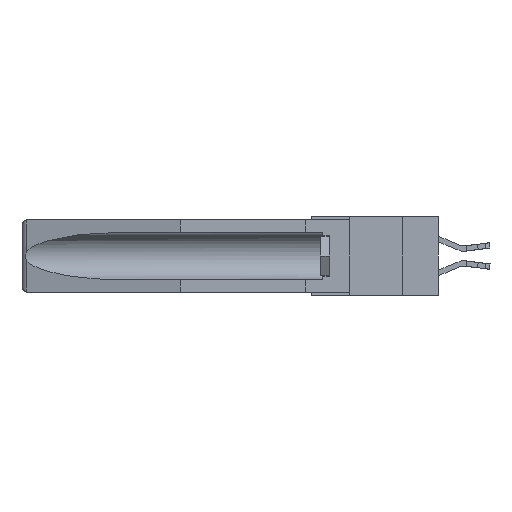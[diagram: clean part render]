
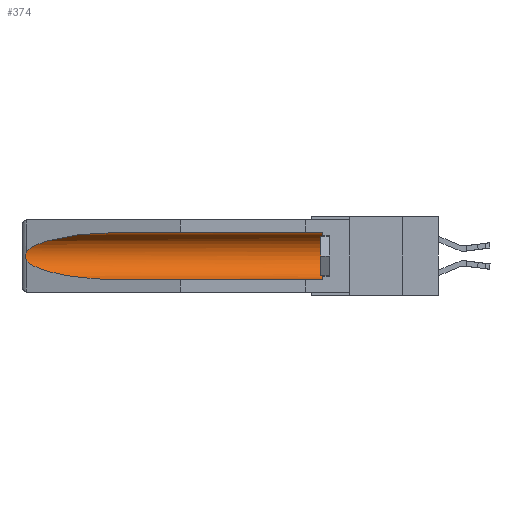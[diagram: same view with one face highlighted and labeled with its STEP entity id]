
A CAD part, left-side view. The second image highlights one B-rep face of the part: STEP entity #374.
In plain terms, the highlighted cylindrical face has radius 2.857 mm (diameter 5.715 mm), a partial arc.
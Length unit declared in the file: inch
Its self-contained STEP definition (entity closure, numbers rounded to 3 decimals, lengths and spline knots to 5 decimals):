
#374 = ADVANCED_FACE ( 'NONE', ( #2719 ), #3018, .F. ) ;
#740 = CARTESIAN_POINT ( 'NONE',  ( 0.155, -0.30754, -0.284 ) ) ;
#839 = CARTESIAN_POINT ( 'NONE',  ( 0.26537, 1.52718, -0.19328 ) ) ;
#1478 = VERTEX_POINT ( 'NONE', #21474 ) ;
#1562 = EDGE_CURVE ( 'NONE', #10676, #8860, #6986, .T. ) ;
#2265 = CARTESIAN_POINT ( 'NONE',  ( 0.26537, 1.52718, -0.14972 ) ) ;
#2579 = CARTESIAN_POINT ( 'NONE',  ( 0.155, 1.07973, -0.284 ) ) ;
#2719 = FACE_OUTER_BOUND ( 'NONE', #22265, .T. ) ;
#2883 = CARTESIAN_POINT ( 'NONE',  ( 0.2673, 1.53269, -0.17917 ) ) ;
#3018 = CYLINDRICAL_SURFACE ( 'NONE', #10121, 0.1125 ) ;
#3127 = CARTESIAN_POINT ( 'NONE',  ( 0.155, 1.07973, -0.284 ) ) ;
#3787 = CIRCLE ( 'NONE', #13490, 0.1125 ) ;
#4490 =( BOUNDED_CURVE ( )  B_SPLINE_CURVE ( 3, ( #14008, #8319, #8402, #23319 ),
 .UNSPECIFIED., .F., .F. ) 
 B_SPLINE_CURVE_WITH_KNOTS ( ( 4, 4 ),
 ( 4.71239, 6.08839 ),
 .UNSPECIFIED. ) 
 CURVE ( )  GEOMETRIC_REPRESENTATION_ITEM ( )  RATIONAL_B_SPLINE_CURVE ( ( 1., 0.848, 0.848, 1. ) ) 
 REPRESENTATION_ITEM ( '' )  );
#4802 = CARTESIAN_POINT ( 'NONE',  ( 0.155, 0.126, -0.059 ) ) ;
#6050 = EDGE_CURVE ( 'NONE', #8860, #18728, #4490, .T. ) ;
#6711 = DIRECTION ( 'NONE',  ( 0., 1., 0. ) ) ;
#6986 = LINE ( 'NONE', #23335, #10484 ) ;
#7245 = EDGE_CURVE ( 'NONE', #14531, #10676, #3787, .T. ) ;
#7285 = VECTOR ( 'NONE', #19203, 39.37008 ) ;
#7473 = DIRECTION ( 'NONE',  ( 0., 1., 0. ) ) ;
#7703 = DIRECTION ( 'NONE',  ( 0., 0., 1. ) ) ;
#8304 = CARTESIAN_POINT ( 'NONE',  ( 0.26654, 1.53092, -0.15636 ) ) ;
#8319 = CARTESIAN_POINT ( 'NONE',  ( 0.21114, 1.30732, -0.059 ) ) ;
#8402 = CARTESIAN_POINT ( 'NONE',  ( 0.25451, 1.48313, -0.09465 ) ) ;
#8860 = VERTEX_POINT ( 'NONE', #21098 ) ;
#9058 = ORIENTED_EDGE ( 'NONE', *, *, #1562, .T. ) ;
#9522 = ORIENTED_EDGE ( 'NONE', *, *, #16842, .T. ) ;
#10023 = CARTESIAN_POINT ( 'NONE',  ( 0.26597, 1.52961, -0.15275 ) ) ;
#10121 = AXIS2_PLACEMENT_3D ( 'NONE', #23621, #7473, #7703 ) ;
#10186 = CARTESIAN_POINT ( 'NONE',  ( 0.25451, 1.48313, -0.24835 ) ) ;
#10333 = CARTESIAN_POINT ( 'NONE',  ( 0.26597, 1.5296, -0.19026 ) ) ;
#10484 = VECTOR ( 'NONE', #6711, 39.37008 ) ;
#10676 = VERTEX_POINT ( 'NONE', #4802 ) ;
#11815 = B_SPLINE_CURVE_WITH_KNOTS ( 'NONE', 3,
 ( #21379, #10023, #8304, #21223, #12161, #13990, #2883, #17662, #10333, #839 ),
 .UNSPECIFIED., .F., .F.,
 ( 4, 2, 2, 2, 4 ),
 ( 0., 0.00029, 0.00058, 0.00087, 0.00117 ),
 .UNSPECIFIED. ) ;
#12161 = CARTESIAN_POINT ( 'NONE',  ( 0.2675, 1.53308, -0.16763 ) ) ;
#13382 = CARTESIAN_POINT ( 'NONE',  ( 0.155, 0.126, -0.284 ) ) ;
#13490 = AXIS2_PLACEMENT_3D ( 'NONE', #14970, #16810, #14818 ) ;
#13832 = CARTESIAN_POINT ( 'NONE',  ( 0.26537, 1.52718, -0.19328 ) ) ;
#13990 = CARTESIAN_POINT ( 'NONE',  ( 0.2675, 1.53308, -0.17534 ) ) ;
#14008 = CARTESIAN_POINT ( 'NONE',  ( 0.155, 1.07973, -0.059 ) ) ;
#14531 = VERTEX_POINT ( 'NONE', #13382 ) ;
#14818 = DIRECTION ( 'NONE',  ( 0., 0., 1. ) ) ;
#14970 = CARTESIAN_POINT ( 'NONE',  ( 0.155, 0.126, -0.1715 ) ) ;
#15400 = ORIENTED_EDGE ( 'NONE', *, *, #6050, .T. ) ;
#15516 = EDGE_CURVE ( 'NONE', #1478, #20900, #20309, .T. ) ;
#15784 = CARTESIAN_POINT ( 'NONE',  ( 0.21114, 1.30732, -0.284 ) ) ;
#16810 = DIRECTION ( 'NONE',  ( 0., -1., 0. ) ) ;
#16842 = EDGE_CURVE ( 'NONE', #18728, #1478, #11815, .T. ) ;
#17662 = CARTESIAN_POINT ( 'NONE',  ( 0.26655, 1.53094, -0.18657 ) ) ;
#17668 = LINE ( 'NONE', #740, #7285 ) ;
#18728 = VERTEX_POINT ( 'NONE', #2265 ) ;
#19203 = DIRECTION ( 'NONE',  ( 0., 1., 0. ) ) ;
#19417 = ORIENTED_EDGE ( 'NONE', *, *, #15516, .T. ) ;
#19816 = ORIENTED_EDGE ( 'NONE', *, *, #7245, .T. ) ;
#20309 =( BOUNDED_CURVE ( )  B_SPLINE_CURVE ( 3, ( #13832, #10186, #15784, #2579 ),
 .UNSPECIFIED., .F., .F. ) 
 B_SPLINE_CURVE_WITH_KNOTS ( ( 4, 4 ),
 ( 0.1948, 1.5708 ),
 .UNSPECIFIED. ) 
 CURVE ( )  GEOMETRIC_REPRESENTATION_ITEM ( )  RATIONAL_B_SPLINE_CURVE ( ( 1., 0.848, 0.848, 1. ) ) 
 REPRESENTATION_ITEM ( '' )  );
#20380 = EDGE_CURVE ( 'NONE', #14531, #20900, #17668, .T. ) ;
#20900 = VERTEX_POINT ( 'NONE', #3127 ) ;
#21098 = CARTESIAN_POINT ( 'NONE',  ( 0.155, 1.07973, -0.059 ) ) ;
#21223 = CARTESIAN_POINT ( 'NONE',  ( 0.2673, 1.5327, -0.16383 ) ) ;
#21379 = CARTESIAN_POINT ( 'NONE',  ( 0.26537, 1.52718, -0.14972 ) ) ;
#21474 = CARTESIAN_POINT ( 'NONE',  ( 0.26537, 1.52718, -0.19328 ) ) ;
#21741 = ORIENTED_EDGE ( 'NONE', *, *, #20380, .F. ) ;
#22265 = EDGE_LOOP ( 'NONE', ( #15400, #9522, #19417, #21741, #19816, #9058 ) ) ;
#23319 = CARTESIAN_POINT ( 'NONE',  ( 0.26537, 1.52718, -0.14972 ) ) ;
#23335 = CARTESIAN_POINT ( 'NONE',  ( 0.155, -0.30754, -0.059 ) ) ;
#23621 = CARTESIAN_POINT ( 'NONE',  ( 0.155, -0.30754, -0.1715 ) ) ;
